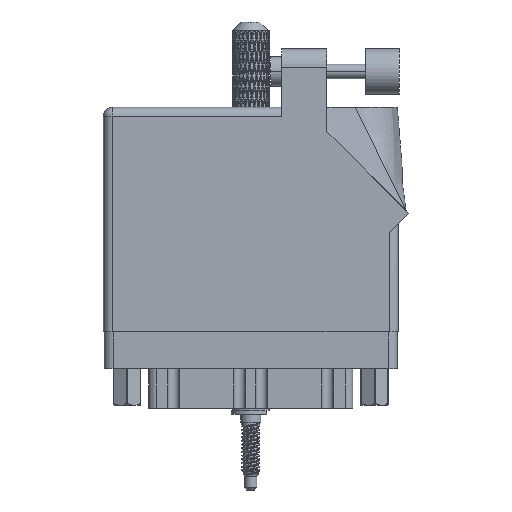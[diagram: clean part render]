
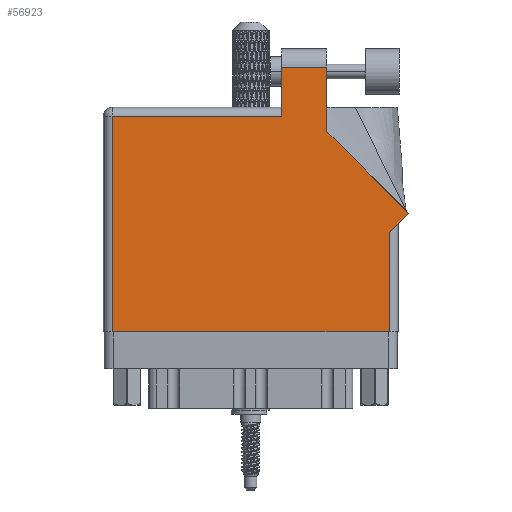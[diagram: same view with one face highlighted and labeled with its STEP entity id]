
A CAD part, front view. The second image highlights one B-rep face of the part: STEP entity #56923.
In plain terms, the highlighted face is planar.
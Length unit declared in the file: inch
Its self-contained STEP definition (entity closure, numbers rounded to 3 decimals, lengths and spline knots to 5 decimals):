
#1993 = ORIENTED_EDGE ( 'NONE', *, *, #109333, .T. ) ;
#2315 = VERTEX_POINT ( 'NONE', #64408 ) ;
#2932 = VECTOR ( 'NONE', #37450, 39.37008 ) ;
#2957 = EDGE_CURVE ( 'NONE', #97892, #91978, #62468, .T. ) ;
#3222 = CARTESIAN_POINT ( 'NONE',  ( 1.217, 1.805, 0. ) ) ;
#3354 = LINE ( 'NONE', #13670, #41617 ) ;
#3653 = LINE ( 'NONE', #48277, #2932 ) ;
#4067 = VECTOR ( 'NONE', #98474, 39.37008 ) ;
#6205 = DIRECTION ( 'NONE',  ( 0., 0., -1. ) ) ;
#6306 = EDGE_LOOP ( 'NONE', ( #62607, #42705, #1993, #63769, #12776, #62693, #86867, #103275, #45996 ) ) ;
#7863 = VERTEX_POINT ( 'NONE', #64819 ) ;
#7958 = VECTOR ( 'NONE', #92850, 39.37008 ) ;
#9104 = CARTESIAN_POINT ( 'NONE',  ( 1.948, 0., 0. ) ) ;
#12776 = ORIENTED_EDGE ( 'NONE', *, *, #75003, .T. ) ;
#13525 = LINE ( 'NONE', #102200, #57295 ) ;
#13670 = CARTESIAN_POINT ( 'NONE',  ( 1.948, 0.737, 0. ) ) ;
#20003 = CARTESIAN_POINT ( 'NONE',  ( 2.08071, 0.80771, 0. ) ) ;
#21106 = DIRECTION ( 'NONE',  ( 0., 1., 0. ) ) ;
#22713 = VECTOR ( 'NONE', #83637, 39.37008 ) ;
#28610 = VERTEX_POINT ( 'NONE', #9104 ) ;
#30113 = VERTEX_POINT ( 'NONE', #33511 ) ;
#31274 = DIRECTION ( 'NONE',  ( -1., 0., 0. ) ) ;
#33511 = CARTESIAN_POINT ( 'NONE',  ( 1.217, 1.805, 0. ) ) ;
#36407 = VECTOR ( 'NONE', #31274, 39.37008 ) ;
#37450 = DIRECTION ( 'NONE',  ( -1., 0., 0. ) ) ;
#40513 = CARTESIAN_POINT ( 'NONE',  ( 0.062, 0., 0. ) ) ;
#41617 = VECTOR ( 'NONE', #21106, 39.37008 ) ;
#42705 = ORIENTED_EDGE ( 'NONE', *, *, #47363, .T. ) ;
#45280 = CARTESIAN_POINT ( 'NONE',  ( 2.01, 0.737, 0. ) ) ;
#45996 = ORIENTED_EDGE ( 'NONE', *, *, #74211, .T. ) ;
#46957 = EDGE_CURVE ( 'NONE', #7863, #2315, #67132, .T. ) ;
#47363 = EDGE_CURVE ( 'NONE', #2315, #30113, #81626, .T. ) ;
#48277 = CARTESIAN_POINT ( 'NONE',  ( 0., 1.468, 0. ) ) ;
#49975 = DIRECTION ( 'NONE',  ( 0., 1., 0. ) ) ;
#52768 = VECTOR ( 'NONE', #49975, 39.37008 ) ;
#54216 = VECTOR ( 'NONE', #106730, 39.37008 ) ;
#56286 = LINE ( 'NONE', #93417, #7958 ) ;
#56923 = ADVANCED_FACE ( 'NONE', ( #110388 ), #69531, .F. ) ;
#57295 = VECTOR ( 'NONE', #110237, 39.37008 ) ;
#58291 = DIRECTION ( 'NONE',  ( -1., 0., 0. ) ) ;
#58560 = CARTESIAN_POINT ( 'NONE',  ( 1.524, 1.36442, 0. ) ) ;
#62468 = LINE ( 'NONE', #45280, #4067 ) ;
#62607 = ORIENTED_EDGE ( 'NONE', *, *, #46957, .T. ) ;
#62693 = ORIENTED_EDGE ( 'NONE', *, *, #99805, .T. ) ;
#63769 = ORIENTED_EDGE ( 'NONE', *, *, #85039, .T. ) ;
#64408 = CARTESIAN_POINT ( 'NONE',  ( 1.524, 1.805, 0. ) ) ;
#64819 = CARTESIAN_POINT ( 'NONE',  ( 1.524, 1.36442, 0. ) ) ;
#65039 = VERTEX_POINT ( 'NONE', #108445 ) ;
#67132 = LINE ( 'NONE', #58560, #52768 ) ;
#69531 = PLANE ( 'NONE',  #88542 ) ;
#70671 = LINE ( 'NONE', #71788, #54216 ) ;
#71788 = CARTESIAN_POINT ( 'NONE',  ( 1.217, 1.53, 0. ) ) ;
#73535 = VERTEX_POINT ( 'NONE', #40513 ) ;
#74143 = CARTESIAN_POINT ( 'NONE',  ( 0.062, 1.468, 0. ) ) ;
#74211 = EDGE_CURVE ( 'NONE', #91978, #7863, #56286, .T. ) ;
#75003 = EDGE_CURVE ( 'NONE', #91631, #73535, #13525, .T. ) ;
#81374 = CARTESIAN_POINT ( 'NONE',  ( 0., 0., 0. ) ) ;
#81626 = LINE ( 'NONE', #3222, #36407 ) ;
#83637 = DIRECTION ( 'NONE',  ( 1., 0., 0. ) ) ;
#84407 = EDGE_CURVE ( 'NONE', #28610, #97892, #3354, .T. ) ;
#85039 = EDGE_CURVE ( 'NONE', #65039, #91631, #3653, .T. ) ;
#86867 = ORIENTED_EDGE ( 'NONE', *, *, #84407, .T. ) ;
#88542 = AXIS2_PLACEMENT_3D ( 'NONE', #101785, #6205, #58291 ) ;
#91631 = VERTEX_POINT ( 'NONE', #74143 ) ;
#91978 = VERTEX_POINT ( 'NONE', #20003 ) ;
#92850 = DIRECTION ( 'NONE',  ( -0.707, 0.707, 0. ) ) ;
#93417 = CARTESIAN_POINT ( 'NONE',  ( 2.08071, 0.80771, 0. ) ) ;
#96208 = CARTESIAN_POINT ( 'NONE',  ( 1.948, 0.675, 0. ) ) ;
#97892 = VERTEX_POINT ( 'NONE', #96208 ) ;
#98474 = DIRECTION ( 'NONE',  ( 0.707, 0.707, 0. ) ) ;
#98561 = LINE ( 'NONE', #81374, #22713 ) ;
#99805 = EDGE_CURVE ( 'NONE', #73535, #28610, #98561, .T. ) ;
#101785 = CARTESIAN_POINT ( 'NONE',  ( 0., 1.53, 0. ) ) ;
#102200 = CARTESIAN_POINT ( 'NONE',  ( 0.062, 0., 0. ) ) ;
#103275 = ORIENTED_EDGE ( 'NONE', *, *, #2957, .T. ) ;
#106730 = DIRECTION ( 'NONE',  ( 0., -1., 0. ) ) ;
#108445 = CARTESIAN_POINT ( 'NONE',  ( 1.217, 1.468, 0. ) ) ;
#109333 = EDGE_CURVE ( 'NONE', #30113, #65039, #70671, .T. ) ;
#110237 = DIRECTION ( 'NONE',  ( 0., -1., 0. ) ) ;
#110388 = FACE_OUTER_BOUND ( 'NONE', #6306, .T. ) ;
